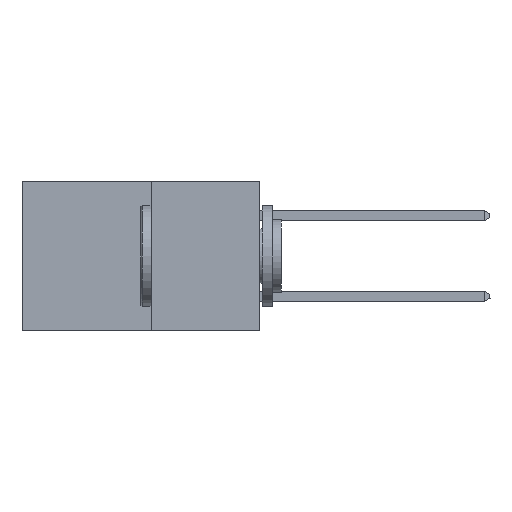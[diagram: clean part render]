
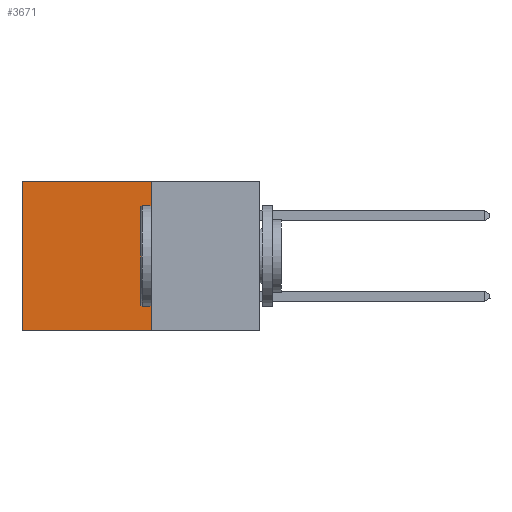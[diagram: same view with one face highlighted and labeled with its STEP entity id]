
A CAD part, left-side view. The second image highlights one B-rep face of the part: STEP entity #3671.
In plain terms, the highlighted planar face has unit normal (-1, 0, 0).
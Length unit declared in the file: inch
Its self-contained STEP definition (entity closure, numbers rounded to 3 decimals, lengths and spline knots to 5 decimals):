
#924 = ORIENTED_EDGE ( 'NONE', *, *, #12758, .F. ) ;
#1406 = LINE ( 'NONE', #15866, #5619 ) ;
#2584 = VERTEX_POINT ( 'NONE', #25836 ) ;
#2817 = VECTOR ( 'NONE', #17725, 39.37008 ) ;
#2945 = ORIENTED_EDGE ( 'NONE', *, *, #4846, .T. ) ;
#3671 = ADVANCED_FACE ( 'NONE', ( #18041 ), #6889, .F. ) ;
#3685 = DIRECTION ( 'NONE',  ( 0., 1., 0. ) ) ;
#3823 = CARTESIAN_POINT ( 'NONE',  ( 0.277, 0.27, 0. ) ) ;
#3826 = EDGE_CURVE ( 'NONE', #2584, #7360, #19631, .T. ) ;
#4846 = EDGE_CURVE ( 'NONE', #7360, #24799, #8346, .T. ) ;
#5619 = VECTOR ( 'NONE', #11838, 39.37008 ) ;
#5646 = CARTESIAN_POINT ( 'NONE',  ( 0.277, 0.59, -0.37 ) ) ;
#6698 = DIRECTION ( 'NONE',  ( 0., 0., -1. ) ) ;
#6741 = DIRECTION ( 'NONE',  ( 1., 0., 0. ) ) ;
#6889 = PLANE ( 'NONE',  #24337 ) ;
#6923 = CARTESIAN_POINT ( 'NONE',  ( 0.277, 0.27, -0.37 ) ) ;
#7360 = VERTEX_POINT ( 'NONE', #23287 ) ;
#8346 = LINE ( 'NONE', #18591, #2817 ) ;
#10275 = ORIENTED_EDGE ( 'NONE', *, *, #14578, .F. ) ;
#11838 = DIRECTION ( 'NONE',  ( 0., 1., 0. ) ) ;
#12758 = EDGE_CURVE ( 'NONE', #18113, #24799, #1406, .T. ) ;
#13591 = VECTOR ( 'NONE', #25454, 39.37008 ) ;
#14180 = VECTOR ( 'NONE', #3685, 39.37008 ) ;
#14578 = EDGE_CURVE ( 'NONE', #2584, #18113, #24356, .T. ) ;
#15866 = CARTESIAN_POINT ( 'NONE',  ( 0.277, 0.27, -0.37 ) ) ;
#17725 = DIRECTION ( 'NONE',  ( 0., 0., -1. ) ) ;
#18041 = FACE_OUTER_BOUND ( 'NONE', #22849, .T. ) ;
#18113 = VERTEX_POINT ( 'NONE', #24199 ) ;
#18591 = CARTESIAN_POINT ( 'NONE',  ( 0.277, 0.59, -0.37 ) ) ;
#19631 = LINE ( 'NONE', #3823, #14180 ) ;
#22849 = EDGE_LOOP ( 'NONE', ( #2945, #924, #10275, #25178 ) ) ;
#23287 = CARTESIAN_POINT ( 'NONE',  ( 0.277, 0.59, 0. ) ) ;
#23426 = CARTESIAN_POINT ( 'NONE',  ( 0.277, 0.27, -0.37 ) ) ;
#24199 = CARTESIAN_POINT ( 'NONE',  ( 0.277, 0.27, -0.37 ) ) ;
#24337 = AXIS2_PLACEMENT_3D ( 'NONE', #6923, #6741, #6698 ) ;
#24356 = LINE ( 'NONE', #23426, #13591 ) ;
#24799 = VERTEX_POINT ( 'NONE', #5646 ) ;
#25178 = ORIENTED_EDGE ( 'NONE', *, *, #3826, .T. ) ;
#25454 = DIRECTION ( 'NONE',  ( 0., 0., -1. ) ) ;
#25836 = CARTESIAN_POINT ( 'NONE',  ( 0.277, 0.27, 0. ) ) ;
